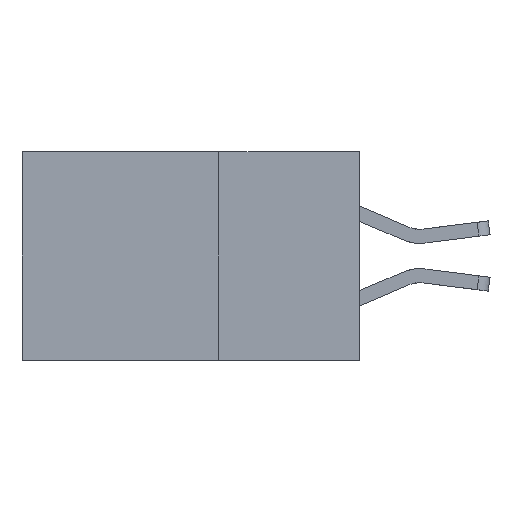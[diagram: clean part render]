
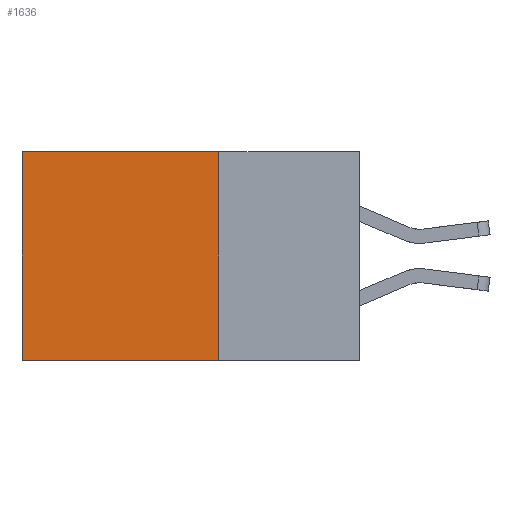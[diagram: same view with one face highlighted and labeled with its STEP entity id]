
A CAD part, left-side view. The second image highlights one B-rep face of the part: STEP entity #1636.
In plain terms, the highlighted planar face has unit normal (-1, 0, 0).
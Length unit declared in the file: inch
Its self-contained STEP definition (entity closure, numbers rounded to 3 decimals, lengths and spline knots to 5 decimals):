
#221 = CARTESIAN_POINT ( 'NONE',  ( 0.2875, 0.25, 0. ) ) ;
#341 = VERTEX_POINT ( 'NONE', #11745 ) ;
#1010 = EDGE_CURVE ( 'NONE', #7214, #7560, #3009, .T. ) ;
#1342 = PLANE ( 'NONE',  #5728 ) ;
#1477 = DIRECTION ( 'NONE',  ( 0., 0., -1. ) ) ;
#1636 = ADVANCED_FACE ( 'NONE', ( #7990 ), #1342, .F. ) ;
#1646 = VECTOR ( 'NONE', #4879, 39.37008 ) ;
#1766 = ORIENTED_EDGE ( 'NONE', *, *, #7301, .F. ) ;
#2165 = VECTOR ( 'NONE', #11062, 39.37008 ) ;
#2217 = CARTESIAN_POINT ( 'NONE',  ( 0.2875, 0.25, 0. ) ) ;
#2310 = DIRECTION ( 'NONE',  ( 0., 1., 0. ) ) ;
#2346 = ORIENTED_EDGE ( 'NONE', *, *, #7586, .F. ) ;
#2563 = CARTESIAN_POINT ( 'NONE',  ( 0.2875, 0.6, 0. ) ) ;
#3009 = LINE ( 'NONE', #2217, #5677 ) ;
#4372 = EDGE_LOOP ( 'NONE', ( #8247, #1766, #2346, #11655 ) ) ;
#4621 = LINE ( 'NONE', #10030, #1646 ) ;
#4879 = DIRECTION ( 'NONE',  ( 0., 1., 0. ) ) ;
#5677 = VECTOR ( 'NONE', #2310, 39.37008 ) ;
#5728 = AXIS2_PLACEMENT_3D ( 'NONE', #221, #12201, #7965 ) ;
#7206 = EDGE_CURVE ( 'NONE', #7560, #7604, #12455, .T. ) ;
#7214 = VERTEX_POINT ( 'NONE', #9340 ) ;
#7301 = EDGE_CURVE ( 'NONE', #341, #7604, #4621, .T. ) ;
#7560 = VERTEX_POINT ( 'NONE', #2563 ) ;
#7586 = EDGE_CURVE ( 'NONE', #7214, #341, #9769, .T. ) ;
#7604 = VERTEX_POINT ( 'NONE', #13131 ) ;
#7965 = DIRECTION ( 'NONE',  ( 0., 0., -1. ) ) ;
#7990 = FACE_OUTER_BOUND ( 'NONE', #4372, .T. ) ;
#8038 = CARTESIAN_POINT ( 'NONE',  ( 0.2875, 0.6, 0. ) ) ;
#8247 = ORIENTED_EDGE ( 'NONE', *, *, #7206, .T. ) ;
#9340 = CARTESIAN_POINT ( 'NONE',  ( 0.2875, 0.25, 0. ) ) ;
#9769 = LINE ( 'NONE', #10056, #12266 ) ;
#10030 = CARTESIAN_POINT ( 'NONE',  ( 0.2875, 0.25, -0.37 ) ) ;
#10056 = CARTESIAN_POINT ( 'NONE',  ( 0.2875, 0.25, 0. ) ) ;
#11062 = DIRECTION ( 'NONE',  ( 0., 0., -1. ) ) ;
#11655 = ORIENTED_EDGE ( 'NONE', *, *, #1010, .T. ) ;
#11745 = CARTESIAN_POINT ( 'NONE',  ( 0.2875, 0.25, -0.37 ) ) ;
#12201 = DIRECTION ( 'NONE',  ( 1., 0., 0. ) ) ;
#12266 = VECTOR ( 'NONE', #1477, 39.37008 ) ;
#12455 = LINE ( 'NONE', #8038, #2165 ) ;
#13131 = CARTESIAN_POINT ( 'NONE',  ( 0.2875, 0.6, -0.37 ) ) ;
